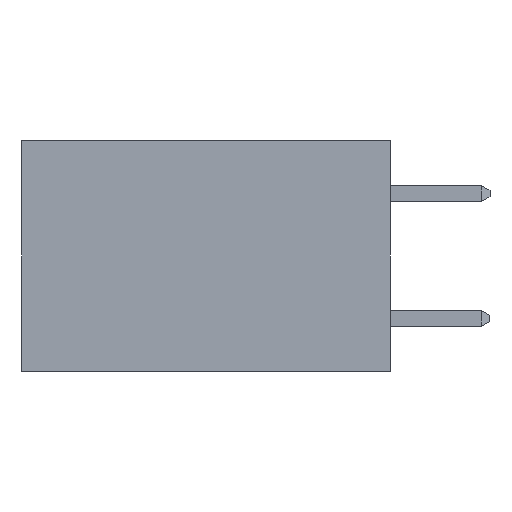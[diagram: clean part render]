
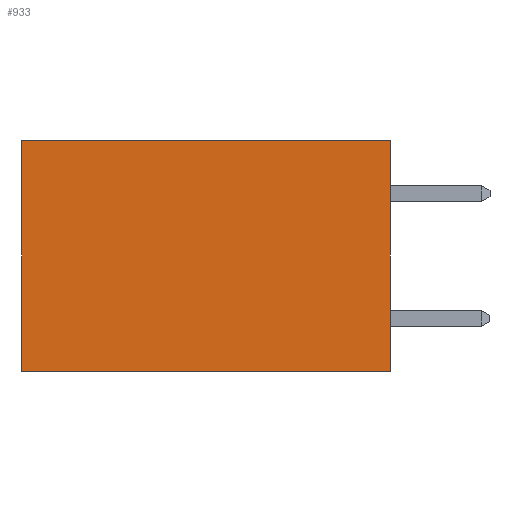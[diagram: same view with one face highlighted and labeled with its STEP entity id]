
A CAD part, left-side view. The second image highlights one B-rep face of the part: STEP entity #933.
In plain terms, the highlighted planar face has unit normal (-1, 0, 0).
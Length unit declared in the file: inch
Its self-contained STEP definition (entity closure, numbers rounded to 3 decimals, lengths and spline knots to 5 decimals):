
#64 = VECTOR ( 'NONE', #1721, 39.37008 ) ;
#121 = LINE ( 'NONE', #2711, #7779 ) ;
#340 = CARTESIAN_POINT ( 'NONE',  ( 0.277, 0., -0.37 ) ) ;
#372 = ORIENTED_EDGE ( 'NONE', *, *, #434, .F. ) ;
#414 = VERTEX_POINT ( 'NONE', #605 ) ;
#434 = EDGE_CURVE ( 'NONE', #414, #2521, #11078, .T. ) ;
#605 = CARTESIAN_POINT ( 'NONE',  ( 0.277, 0., 0. ) ) ;
#632 = CARTESIAN_POINT ( 'NONE',  ( 0.277, 0., 0. ) ) ;
#673 = ORIENTED_EDGE ( 'NONE', *, *, #11935, .T. ) ;
#933 = ADVANCED_FACE ( 'NONE', ( #9629 ), #11259, .F. ) ;
#1721 = DIRECTION ( 'NONE',  ( 0., 0., -1. ) ) ;
#1792 = CARTESIAN_POINT ( 'NONE',  ( 0.277, 0.59, -0.37 ) ) ;
#2346 = CARTESIAN_POINT ( 'NONE',  ( 0.277, 0.59, 0. ) ) ;
#2521 = VERTEX_POINT ( 'NONE', #340 ) ;
#2567 = DIRECTION ( 'NONE',  ( 0., 1., 0. ) ) ;
#2634 = ORIENTED_EDGE ( 'NONE', *, *, #3039, .T. ) ;
#2675 = VERTEX_POINT ( 'NONE', #2346 ) ;
#2681 = DIRECTION ( 'NONE',  ( 0., 1., 0. ) ) ;
#2711 = CARTESIAN_POINT ( 'NONE',  ( 0.277, 0., -0.37 ) ) ;
#3039 = EDGE_CURVE ( 'NONE', #2675, #7685, #7436, .T. ) ;
#6181 = CARTESIAN_POINT ( 'NONE',  ( 0.277, 0., -0.37 ) ) ;
#6371 = EDGE_CURVE ( 'NONE', #2521, #7685, #121, .T. ) ;
#6572 = VECTOR ( 'NONE', #2567, 39.37008 ) ;
#7112 = EDGE_LOOP ( 'NONE', ( #2634, #10267, #372, #673 ) ) ;
#7436 = LINE ( 'NONE', #1792, #64 ) ;
#7521 = DIRECTION ( 'NONE',  ( 1., 0., 0. ) ) ;
#7685 = VERTEX_POINT ( 'NONE', #9585 ) ;
#7779 = VECTOR ( 'NONE', #2681, 39.37008 ) ;
#8582 = VECTOR ( 'NONE', #10398, 39.37008 ) ;
#9148 = LINE ( 'NONE', #632, #6572 ) ;
#9585 = CARTESIAN_POINT ( 'NONE',  ( 0.277, 0.59, -0.37 ) ) ;
#9629 = FACE_OUTER_BOUND ( 'NONE', #7112, .T. ) ;
#10267 = ORIENTED_EDGE ( 'NONE', *, *, #6371, .F. ) ;
#10306 = DIRECTION ( 'NONE',  ( 0., 0., -1. ) ) ;
#10398 = DIRECTION ( 'NONE',  ( 0., 0., -1. ) ) ;
#11078 = LINE ( 'NONE', #6181, #8582 ) ;
#11104 = AXIS2_PLACEMENT_3D ( 'NONE', #11668, #7521, #10306 ) ;
#11259 = PLANE ( 'NONE',  #11104 ) ;
#11668 = CARTESIAN_POINT ( 'NONE',  ( 0.277, 0., -0.37 ) ) ;
#11935 = EDGE_CURVE ( 'NONE', #414, #2675, #9148, .T. ) ;
